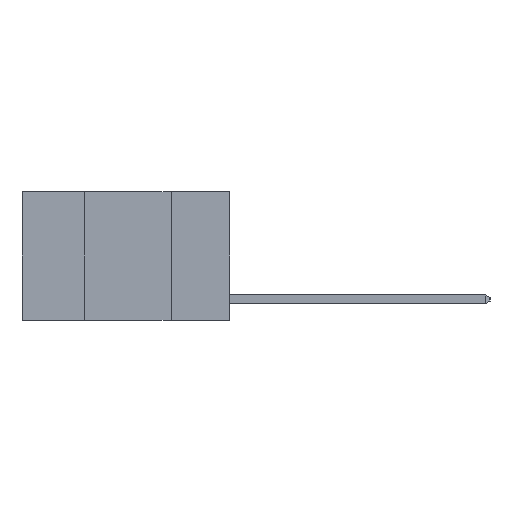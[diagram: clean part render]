
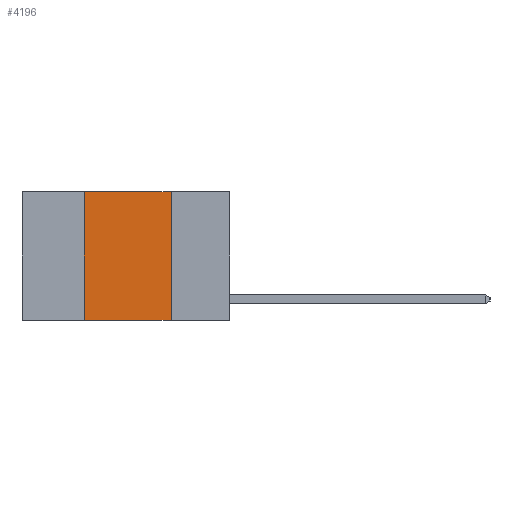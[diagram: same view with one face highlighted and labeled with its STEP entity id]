
A CAD part, left-side view. The second image highlights one B-rep face of the part: STEP entity #4196.
In plain terms, the highlighted planar face has unit normal (-1, 0, 0).
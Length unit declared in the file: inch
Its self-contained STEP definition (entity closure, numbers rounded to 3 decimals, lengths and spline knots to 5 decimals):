
#406 = VECTOR ( 'NONE', #2634, 39.37008 ) ;
#787 = ORIENTED_EDGE ( 'NONE', *, *, #9901, .T. ) ;
#1292 = EDGE_CURVE ( 'NONE', #8937, #7341, #5574, .T. ) ;
#1294 = EDGE_LOOP ( 'NONE', ( #8101, #5219, #6648, #787 ) ) ;
#1332 = EDGE_CURVE ( 'NONE', #9136, #8937, #9201, .T. ) ;
#1854 = CARTESIAN_POINT ( 'NONE',  ( 0., 0.6, -0.37 ) ) ;
#1860 = CARTESIAN_POINT ( 'NONE',  ( 0., 0.6, 0. ) ) ;
#2582 = CARTESIAN_POINT ( 'NONE',  ( 0., 0.17, 0. ) ) ;
#2634 = DIRECTION ( 'NONE',  ( 0., -1., 0. ) ) ;
#2780 = LINE ( 'NONE', #3978, #8896 ) ;
#3263 = FACE_OUTER_BOUND ( 'NONE', #1294, .T. ) ;
#3308 = VECTOR ( 'NONE', #7149, 39.37008 ) ;
#3352 = CARTESIAN_POINT ( 'NONE',  ( 0., 0.17, -0.37 ) ) ;
#3399 = CARTESIAN_POINT ( 'NONE',  ( 0., 0.42, -0.37 ) ) ;
#3911 = CARTESIAN_POINT ( 'NONE',  ( 0., 0.6, 0. ) ) ;
#3943 = DIRECTION ( 'NONE',  ( 0., 0., -1. ) ) ;
#3978 = CARTESIAN_POINT ( 'NONE',  ( 0., 0.42, 0. ) ) ;
#4196 = ADVANCED_FACE ( 'NONE', ( #3263 ), #5454, .F. ) ;
#4223 = EDGE_CURVE ( 'NONE', #6703, #9136, #2780, .T. ) ;
#4479 = LINE ( 'NONE', #1854, #406 ) ;
#5219 = ORIENTED_EDGE ( 'NONE', *, *, #1332, .F. ) ;
#5454 = PLANE ( 'NONE',  #6861 ) ;
#5574 = LINE ( 'NONE', #2582, #3308 ) ;
#5898 = CARTESIAN_POINT ( 'NONE',  ( 0., 0.17, 0. ) ) ;
#6648 = ORIENTED_EDGE ( 'NONE', *, *, #4223, .F. ) ;
#6703 = VERTEX_POINT ( 'NONE', #3399 ) ;
#6861 = AXIS2_PLACEMENT_3D ( 'NONE', #3911, #8536, #3943 ) ;
#7149 = DIRECTION ( 'NONE',  ( 0., 0., -1. ) ) ;
#7341 = VERTEX_POINT ( 'NONE', #3352 ) ;
#7691 = CARTESIAN_POINT ( 'NONE',  ( 0., 0.42, 0. ) ) ;
#7940 = DIRECTION ( 'NONE',  ( 0., -1., 0. ) ) ;
#8101 = ORIENTED_EDGE ( 'NONE', *, *, #1292, .F. ) ;
#8536 = DIRECTION ( 'NONE',  ( 1., 0., 0. ) ) ;
#8575 = DIRECTION ( 'NONE',  ( 0., 0., 1. ) ) ;
#8896 = VECTOR ( 'NONE', #8575, 39.37008 ) ;
#8937 = VERTEX_POINT ( 'NONE', #5898 ) ;
#9136 = VERTEX_POINT ( 'NONE', #7691 ) ;
#9201 = LINE ( 'NONE', #1860, #9441 ) ;
#9441 = VECTOR ( 'NONE', #7940, 39.37008 ) ;
#9901 = EDGE_CURVE ( 'NONE', #6703, #7341, #4479, .T. ) ;
